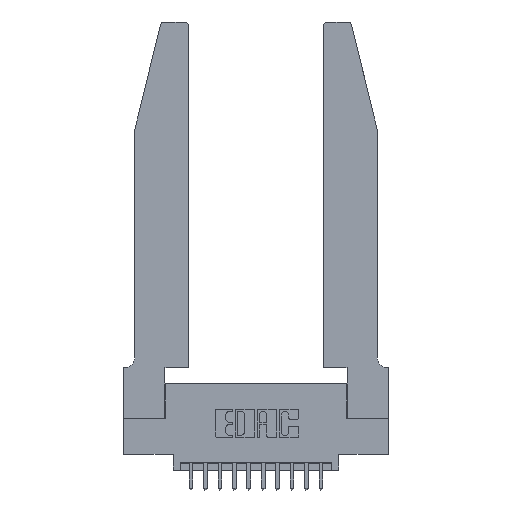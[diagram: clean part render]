
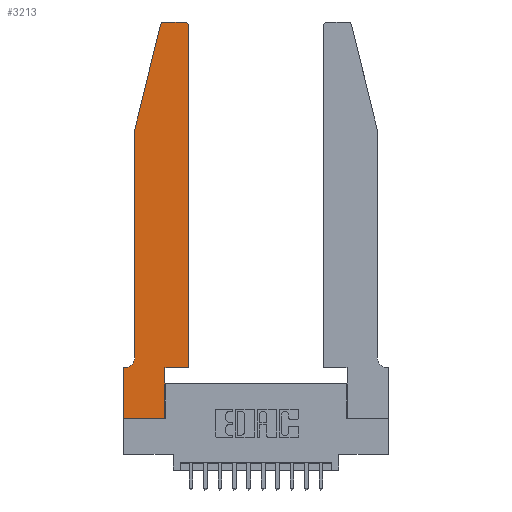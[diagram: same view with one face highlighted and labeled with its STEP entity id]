
A CAD part, top view. The second image highlights one B-rep face of the part: STEP entity #3213.
In plain terms, the highlighted planar face has unit normal (0, 0, 1).
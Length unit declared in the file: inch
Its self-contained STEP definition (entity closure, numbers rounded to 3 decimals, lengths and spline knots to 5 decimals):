
#259 = VECTOR ( 'NONE', #9032, 39.37008 ) ;
#310 = CARTESIAN_POINT ( 'NONE',  ( 0., 0., 0.37 ) ) ;
#420 = DIRECTION ( 'NONE',  ( 0., 0., 1. ) ) ;
#533 = VECTOR ( 'NONE', #12841, 39.37008 ) ;
#579 = DIRECTION ( 'NONE',  ( -0.239, -0.971, 0. ) ) ;
#602 = ORIENTED_EDGE ( 'NONE', *, *, #4404, .T. ) ;
#840 = CARTESIAN_POINT ( 'NONE',  ( 0.4505, 0.35, 0.37 ) ) ;
#921 = CIRCLE ( 'NONE', #4215, 0.07 ) ;
#965 = VERTEX_POINT ( 'NONE', #11126 ) ;
#1010 = CIRCLE ( 'NONE', #13267, 0.03 ) ;
#1049 = LINE ( 'NONE', #14541, #14652 ) ;
#1607 = DIRECTION ( 'NONE',  ( 0., 0., 1. ) ) ;
#1817 = VERTEX_POINT ( 'NONE', #840 ) ;
#1869 = CARTESIAN_POINT ( 'NONE',  ( 0.2865, 0.35, 0.37 ) ) ;
#1946 = CARTESIAN_POINT ( 'NONE',  ( 0.0755, 2., 0.37 ) ) ;
#2169 = VECTOR ( 'NONE', #2391, 39.37008 ) ;
#2284 = LINE ( 'NONE', #310, #15865 ) ;
#2374 = ORIENTED_EDGE ( 'NONE', *, *, #2620, .T. ) ;
#2391 = DIRECTION ( 'NONE',  ( 1., 0., 0. ) ) ;
#2620 = EDGE_CURVE ( 'NONE', #15354, #14553, #15046, .T. ) ;
#2679 = DIRECTION ( 'NONE',  ( 0., 0., -1. ) ) ;
#3194 = EDGE_CURVE ( 'NONE', #965, #4397, #1010, .T. ) ;
#3213 = ADVANCED_FACE ( 'NONE', ( #4199 ), #14723, .T. ) ;
#3829 = VERTEX_POINT ( 'NONE', #12168 ) ;
#4199 = FACE_OUTER_BOUND ( 'NONE', #5278, .T. ) ;
#4212 = EDGE_CURVE ( 'NONE', #14553, #965, #10725, .T. ) ;
#4215 = AXIS2_PLACEMENT_3D ( 'NONE', #10585, #2679, #11915 ) ;
#4249 = ORIENTED_EDGE ( 'NONE', *, *, #6423, .T. ) ;
#4397 = VERTEX_POINT ( 'NONE', #13233 ) ;
#4404 = EDGE_CURVE ( 'NONE', #3829, #10766, #4770, .T. ) ;
#4671 = CARTESIAN_POINT ( 'NONE',  ( 0.0755, 2., 0.37 ) ) ;
#4738 = EDGE_CURVE ( 'NONE', #6504, #4795, #2284, .T. ) ;
#4770 = LINE ( 'NONE', #15851, #11336 ) ;
#4795 = VERTEX_POINT ( 'NONE', #7821 ) ;
#5007 = CARTESIAN_POINT ( 'NONE',  ( 0.2605, 2.75, 0.37 ) ) ;
#5176 = ORIENTED_EDGE ( 'NONE', *, *, #3194, .T. ) ;
#5278 = EDGE_LOOP ( 'NONE', ( #15599, #5176, #16033, #10141, #11590, #602, #6523, #8962, #4249, #13527, #12292, #2374 ) ) ;
#6218 = VERTEX_POINT ( 'NONE', #4671 ) ;
#6423 = EDGE_CURVE ( 'NONE', #4795, #6753, #7418, .T. ) ;
#6504 = VERTEX_POINT ( 'NONE', #13092 ) ;
#6518 = EDGE_CURVE ( 'NONE', #1817, #15354, #9610, .T. ) ;
#6523 = ORIENTED_EDGE ( 'NONE', *, *, #9061, .T. ) ;
#6580 = VECTOR ( 'NONE', #10450, 39.37008 ) ;
#6753 = VERTEX_POINT ( 'NONE', #1869 ) ;
#6936 = CARTESIAN_POINT ( 'NONE',  ( 0.284, 2.72, 0.37 ) ) ;
#7418 = LINE ( 'NONE', #7745, #259 ) ;
#7745 = CARTESIAN_POINT ( 'NONE',  ( 0.2865, 0.35, 0.37 ) ) ;
#7821 = CARTESIAN_POINT ( 'NONE',  ( 0.2865, 0., 0.37 ) ) ;
#8038 = DIRECTION ( 'NONE',  ( -1., 0., 0. ) ) ;
#8241 = DIRECTION ( 'NONE',  ( 1., 0., 0. ) ) ;
#8311 = DIRECTION ( 'NONE',  ( 1., 0., 0. ) ) ;
#8421 = CARTESIAN_POINT ( 'NONE',  ( 0.4205, 2.72, 0.37 ) ) ;
#8557 = VECTOR ( 'NONE', #12132, 39.37008 ) ;
#8569 = EDGE_CURVE ( 'NONE', #6218, #11742, #12057, .T. ) ;
#8962 = ORIENTED_EDGE ( 'NONE', *, *, #4738, .T. ) ;
#9032 = DIRECTION ( 'NONE',  ( 0., 1., 0. ) ) ;
#9061 = EDGE_CURVE ( 'NONE', #10766, #6504, #1049, .T. ) ;
#9244 = CARTESIAN_POINT ( 'NONE',  ( 0., 0.35, 0.37 ) ) ;
#9525 = CARTESIAN_POINT ( 'NONE',  ( 0., 0.35, 0.37 ) ) ;
#9610 = LINE ( 'NONE', #14395, #6580 ) ;
#9719 = DIRECTION ( 'NONE',  ( 1., 0., 0. ) ) ;
#10137 = EDGE_CURVE ( 'NONE', #11742, #3829, #921, .T. ) ;
#10141 = ORIENTED_EDGE ( 'NONE', *, *, #8569, .T. ) ;
#10226 = CARTESIAN_POINT ( 'NONE',  ( 0.0755, 0.42, 0.37 ) ) ;
#10300 = CARTESIAN_POINT ( 'NONE',  ( 0.4505, 0.35, 0.37 ) ) ;
#10450 = DIRECTION ( 'NONE',  ( 0., 1., 0. ) ) ;
#10455 = EDGE_CURVE ( 'NONE', #4397, #6218, #10458, .T. ) ;
#10458 = LINE ( 'NONE', #1946, #13521 ) ;
#10585 = CARTESIAN_POINT ( 'NONE',  ( 0.0055, 0.42, 0.37 ) ) ;
#10725 = LINE ( 'NONE', #5007, #533 ) ;
#10766 = VERTEX_POINT ( 'NONE', #9244 ) ;
#10854 = DIRECTION ( 'NONE',  ( 1., 0., 0. ) ) ;
#11046 = EDGE_CURVE ( 'NONE', #6753, #1817, #12286, .T. ) ;
#11126 = CARTESIAN_POINT ( 'NONE',  ( 0.284, 2.75, 0.37 ) ) ;
#11336 = VECTOR ( 'NONE', #8038, 39.37008 ) ;
#11590 = ORIENTED_EDGE ( 'NONE', *, *, #10137, .T. ) ;
#11742 = VERTEX_POINT ( 'NONE', #10226 ) ;
#11915 = DIRECTION ( 'NONE',  ( -1., 0., 0. ) ) ;
#12057 = LINE ( 'NONE', #13383, #8557 ) ;
#12132 = DIRECTION ( 'NONE',  ( 0., -1., 0. ) ) ;
#12168 = CARTESIAN_POINT ( 'NONE',  ( 0.0055, 0.35, 0.37 ) ) ;
#12286 = LINE ( 'NONE', #10300, #2169 ) ;
#12292 = ORIENTED_EDGE ( 'NONE', *, *, #6518, .T. ) ;
#12841 = DIRECTION ( 'NONE',  ( -1., 0., 0. ) ) ;
#12989 = CARTESIAN_POINT ( 'NONE',  ( 0.4205, 2.75, 0.37 ) ) ;
#13045 = AXIS2_PLACEMENT_3D ( 'NONE', #8421, #420, #9719 ) ;
#13092 = CARTESIAN_POINT ( 'NONE',  ( 0., 0., 0.37 ) ) ;
#13233 = CARTESIAN_POINT ( 'NONE',  ( 0.25487, 2.72718, 0.37 ) ) ;
#13267 = AXIS2_PLACEMENT_3D ( 'NONE', #6936, #16042, #8241 ) ;
#13305 = DIRECTION ( 'NONE',  ( 0., -1., 0. ) ) ;
#13383 = CARTESIAN_POINT ( 'NONE',  ( 0.0755, 2., 0.37 ) ) ;
#13418 = CARTESIAN_POINT ( 'NONE',  ( 0.4505, 2.72, 0.37 ) ) ;
#13521 = VECTOR ( 'NONE', #579, 39.37008 ) ;
#13527 = ORIENTED_EDGE ( 'NONE', *, *, #11046, .T. ) ;
#14395 = CARTESIAN_POINT ( 'NONE',  ( 0.4505, 0.35, 0.37 ) ) ;
#14541 = CARTESIAN_POINT ( 'NONE',  ( 0., 0., 0.37 ) ) ;
#14553 = VERTEX_POINT ( 'NONE', #12989 ) ;
#14652 = VECTOR ( 'NONE', #13305, 39.37008 ) ;
#14723 = PLANE ( 'NONE',  #16729 ) ;
#15046 = CIRCLE ( 'NONE', #13045, 0.03 ) ;
#15354 = VERTEX_POINT ( 'NONE', #13418 ) ;
#15599 = ORIENTED_EDGE ( 'NONE', *, *, #4212, .T. ) ;
#15851 = CARTESIAN_POINT ( 'NONE',  ( 0.0755, 0.35, 0.37 ) ) ;
#15865 = VECTOR ( 'NONE', #8311, 39.37008 ) ;
#16033 = ORIENTED_EDGE ( 'NONE', *, *, #10455, .T. ) ;
#16042 = DIRECTION ( 'NONE',  ( 0., 0., 1. ) ) ;
#16729 = AXIS2_PLACEMENT_3D ( 'NONE', #9525, #1607, #10854 ) ;
